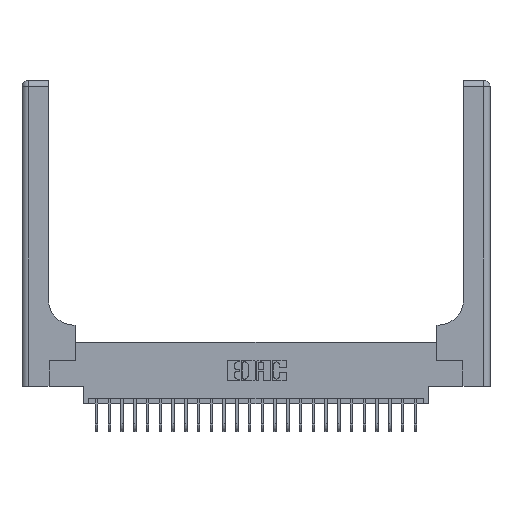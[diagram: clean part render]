
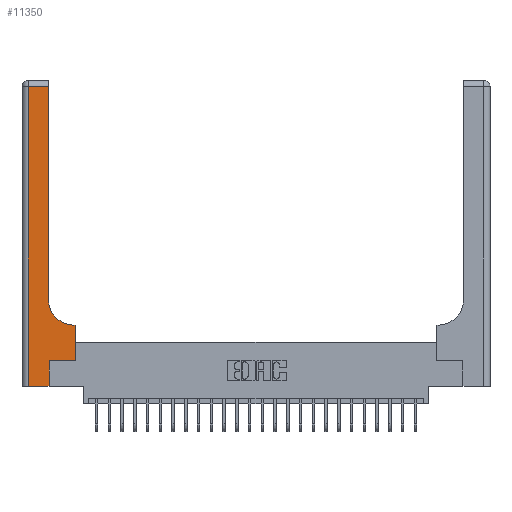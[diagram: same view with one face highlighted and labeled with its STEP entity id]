
A CAD part, top view. The second image highlights one B-rep face of the part: STEP entity #11350.
In plain terms, the highlighted planar face has unit normal (0, 0, 1).
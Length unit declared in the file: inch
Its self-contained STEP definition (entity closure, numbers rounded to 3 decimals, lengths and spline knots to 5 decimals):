
#125 = VECTOR ( 'NONE', #26143, 39.37008 ) ;
#1434 = CARTESIAN_POINT ( 'NONE',  ( 0.265, 0.25, 0.37 ) ) ;
#2308 = AXIS2_PLACEMENT_3D ( 'NONE', #19262, #16729, #22783 ) ;
#2584 = DIRECTION ( 'NONE',  ( -1., 0., 0. ) ) ;
#3247 = AXIS2_PLACEMENT_3D ( 'NONE', #12370, #6130, #4263 ) ;
#3614 = LINE ( 'NONE', #23590, #20038 ) ;
#4011 = EDGE_CURVE ( 'NONE', #6382, #5520, #6255, .T. ) ;
#4209 = LINE ( 'NONE', #6356, #20985 ) ;
#4263 = DIRECTION ( 'NONE',  ( 1., 0., 0. ) ) ;
#4543 = CARTESIAN_POINT ( 'NONE',  ( 0.06, 0., 0.37 ) ) ;
#5227 = EDGE_CURVE ( 'NONE', #5520, #5778, #6195, .T. ) ;
#5520 = VERTEX_POINT ( 'NONE', #10090 ) ;
#5610 = LINE ( 'NONE', #1434, #125 ) ;
#5635 = DIRECTION ( 'NONE',  ( 0., 1., 0. ) ) ;
#5778 = VERTEX_POINT ( 'NONE', #25743 ) ;
#6101 = ORIENTED_EDGE ( 'NONE', *, *, #4011, .T. ) ;
#6130 = DIRECTION ( 'NONE',  ( 0., 0., -1. ) ) ;
#6195 = LINE ( 'NONE', #12961, #14289 ) ;
#6255 = LINE ( 'NONE', #8700, #11210 ) ;
#6356 = CARTESIAN_POINT ( 'NONE',  ( 0., 2.94, 0.37 ) ) ;
#6382 = VERTEX_POINT ( 'NONE', #7747 ) ;
#6497 = DIRECTION ( 'NONE',  ( -1., 0., 0. ) ) ;
#6520 = CARTESIAN_POINT ( 'NONE',  ( 0.265, 0.25, 0.37 ) ) ;
#6975 = CARTESIAN_POINT ( 'NONE',  ( 0.26, 2.94, 0.37 ) ) ;
#7072 = ORIENTED_EDGE ( 'NONE', *, *, #13723, .T. ) ;
#7747 = CARTESIAN_POINT ( 'NONE',  ( 0.528, 0.25, 0.37 ) ) ;
#8107 = CARTESIAN_POINT ( 'NONE',  ( 0.06, 2.94, 0.37 ) ) ;
#8482 = PLANE ( 'NONE',  #2308 ) ;
#8700 = CARTESIAN_POINT ( 'NONE',  ( 0.528, 0.25, 0.37 ) ) ;
#8941 = EDGE_CURVE ( 'NONE', #16960, #15470, #3614, .T. ) ;
#9946 = VERTEX_POINT ( 'NONE', #18196 ) ;
#10080 = LINE ( 'NONE', #26566, #22303 ) ;
#10090 = CARTESIAN_POINT ( 'NONE',  ( 0.528, 0.6, 0.37 ) ) ;
#10186 = EDGE_CURVE ( 'NONE', #25663, #16960, #17363, .T. ) ;
#10937 = VERTEX_POINT ( 'NONE', #8107 ) ;
#11210 = VECTOR ( 'NONE', #16675, 39.37008 ) ;
#11350 = ADVANCED_FACE ( 'NONE', ( #20779 ), #8482, .F. ) ;
#11403 = DIRECTION ( 'NONE',  ( 1., 0., 0. ) ) ;
#12016 = ORIENTED_EDGE ( 'NONE', *, *, #10186, .T. ) ;
#12207 = ORIENTED_EDGE ( 'NONE', *, *, #23851, .T. ) ;
#12370 = CARTESIAN_POINT ( 'NONE',  ( 0.51, 0.85, 0.37 ) ) ;
#12961 = CARTESIAN_POINT ( 'NONE',  ( 0.26, 0.6, 0.37 ) ) ;
#13723 = EDGE_CURVE ( 'NONE', #5778, #9946, #26524, .T. ) ;
#14289 = VECTOR ( 'NONE', #2584, 39.37008 ) ;
#14560 = VECTOR ( 'NONE', #16841, 39.37008 ) ;
#14994 = ORIENTED_EDGE ( 'NONE', *, *, #5227, .T. ) ;
#15036 = EDGE_CURVE ( 'NONE', #10937, #25663, #20878, .T. ) ;
#15470 = VERTEX_POINT ( 'NONE', #6520 ) ;
#16675 = DIRECTION ( 'NONE',  ( 0., 1., 0. ) ) ;
#16729 = DIRECTION ( 'NONE',  ( 0., 0., -1. ) ) ;
#16841 = DIRECTION ( 'NONE',  ( 0., -1., 0. ) ) ;
#16960 = VERTEX_POINT ( 'NONE', #24195 ) ;
#17363 = LINE ( 'NONE', #25572, #25854 ) ;
#18196 = CARTESIAN_POINT ( 'NONE',  ( 0.26, 0.85, 0.37 ) ) ;
#18859 = CARTESIAN_POINT ( 'NONE',  ( 0.06, 3., 0.37 ) ) ;
#19262 = CARTESIAN_POINT ( 'NONE',  ( 0., 3., 0.37 ) ) ;
#19964 = EDGE_CURVE ( 'NONE', #15470, #6382, #5610, .T. ) ;
#20038 = VECTOR ( 'NONE', #26158, 39.37008 ) ;
#20779 = FACE_OUTER_BOUND ( 'NONE', #25980, .T. ) ;
#20878 = LINE ( 'NONE', #18859, #14560 ) ;
#20985 = VECTOR ( 'NONE', #6497, 39.37008 ) ;
#21588 = ORIENTED_EDGE ( 'NONE', *, *, #25583, .T. ) ;
#22303 = VECTOR ( 'NONE', #5635, 39.37008 ) ;
#22783 = DIRECTION ( 'NONE',  ( -1., 0., 0. ) ) ;
#23250 = VERTEX_POINT ( 'NONE', #6975 ) ;
#23590 = CARTESIAN_POINT ( 'NONE',  ( 0.265, 0., 0.37 ) ) ;
#23812 = ORIENTED_EDGE ( 'NONE', *, *, #19964, .T. ) ;
#23851 = EDGE_CURVE ( 'NONE', #23250, #10937, #4209, .T. ) ;
#24195 = CARTESIAN_POINT ( 'NONE',  ( 0.265, 0., 0.37 ) ) ;
#24770 = ORIENTED_EDGE ( 'NONE', *, *, #8941, .T. ) ;
#24824 = ORIENTED_EDGE ( 'NONE', *, *, #15036, .T. ) ;
#25572 = CARTESIAN_POINT ( 'NONE',  ( 0., 0., 0.37 ) ) ;
#25583 = EDGE_CURVE ( 'NONE', #9946, #23250, #10080, .T. ) ;
#25663 = VERTEX_POINT ( 'NONE', #4543 ) ;
#25743 = CARTESIAN_POINT ( 'NONE',  ( 0.51, 0.6, 0.37 ) ) ;
#25854 = VECTOR ( 'NONE', #11403, 39.37008 ) ;
#25980 = EDGE_LOOP ( 'NONE', ( #21588, #12207, #24824, #12016, #24770, #23812, #6101, #14994, #7072 ) ) ;
#26143 = DIRECTION ( 'NONE',  ( 1., 0., 0. ) ) ;
#26158 = DIRECTION ( 'NONE',  ( 0., 1., 0. ) ) ;
#26524 = CIRCLE ( 'NONE', #3247, 0.25 ) ;
#26566 = CARTESIAN_POINT ( 'NONE',  ( 0.26, 3., 0.37 ) ) ;
